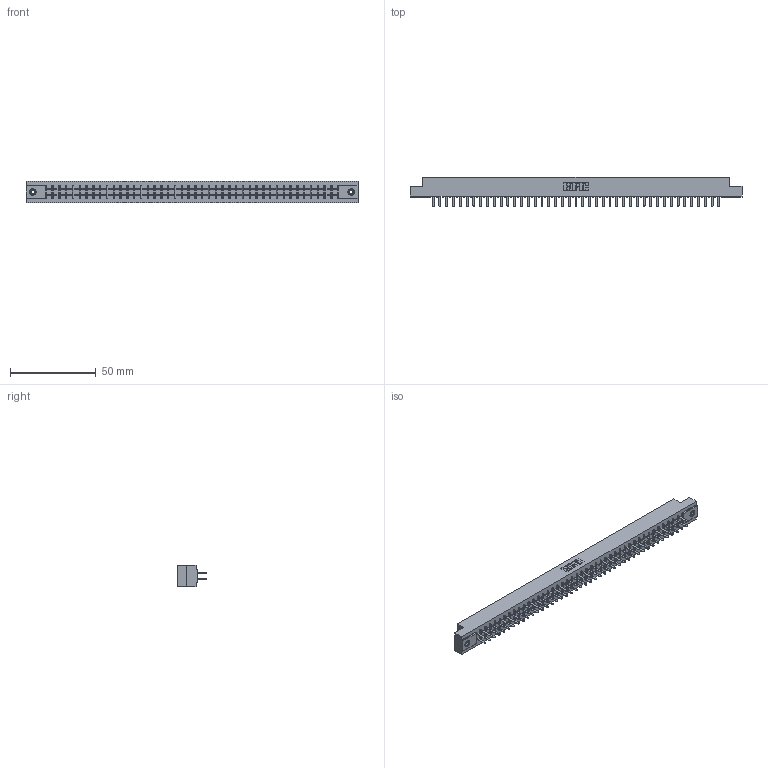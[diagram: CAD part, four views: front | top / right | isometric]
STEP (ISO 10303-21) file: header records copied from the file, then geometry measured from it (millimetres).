
FILE_DESCRIPTION (( 'STEP AP203' ), '1' );
FILE_NAME ('305-086-520-208.STEP', '2019-09-10T12:45:30', ( '' ), ( '' ), 'SwSTEP 2.0', 'SolidWorks 2016', '' );
FILE_SCHEMA (( 'CONFIG_CONTROL_DESIGN' ));
Length unit declared in the file: inch
Products named in the file (4): 345-250-001_345-250-003-102; 305 Part_.156 Dia; 305-290-001_520; 305-086-520-208
Assembly tree (89 placements, depth 2):
  305-086-520-208
    305 Part_.156 Dia
    305-290-001_520  x86
    345-250-001_345-250-003-102  x2
Bounding box: 193.4 x 17.09 x 12.7 mm (x, y, z)
Volume: 20161.1 mm3; surface area: 25773.8 mm2
Topology: 89 solids, 89 shells, 4132 faces, 11761 edges, 7602 vertices
Faces by surface type: plane 2422, cylinder 1522, sphere 172, cone 12, torus 4
Entity records: 47501 total; most frequent: CARTESIAN_POINT 7842, ORIENTED_EDGE 7778, DIRECTION 7595, EDGE_CURVE 3889, LINE 3145, VECTOR 3145, VERTEX_POINT 2472, AXIS2_PLACEMENT_3D 2225
